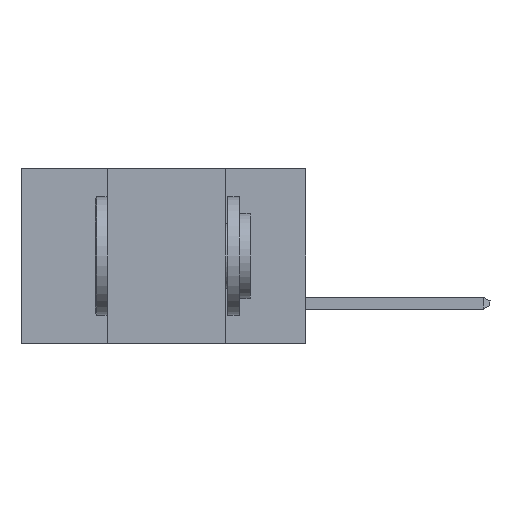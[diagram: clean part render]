
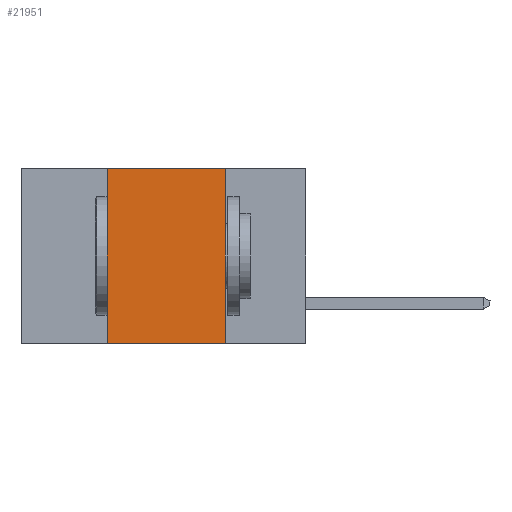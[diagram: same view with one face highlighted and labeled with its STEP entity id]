
A CAD part, left-side view. The second image highlights one B-rep face of the part: STEP entity #21951.
In plain terms, the highlighted planar face has unit normal (-1, 0, 0).
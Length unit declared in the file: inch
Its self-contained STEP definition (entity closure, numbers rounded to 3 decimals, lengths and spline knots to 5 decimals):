
#622 = LINE ( 'NONE', #13256, #5973 ) ;
#3241 = CARTESIAN_POINT ( 'NONE',  ( 0., 0.6, -0.37 ) ) ;
#3280 = EDGE_CURVE ( 'NONE', #24611, #7373, #12283, .T. ) ;
#3740 = CARTESIAN_POINT ( 'NONE',  ( 0., 0.42, -0.37 ) ) ;
#4066 = ORIENTED_EDGE ( 'NONE', *, *, #8670, .T. ) ;
#4547 = CARTESIAN_POINT ( 'NONE',  ( 0., 0.6, 0. ) ) ;
#5973 = VECTOR ( 'NONE', #11085, 39.37008 ) ;
#7336 = VECTOR ( 'NONE', #20811, 39.37008 ) ;
#7368 = CARTESIAN_POINT ( 'NONE',  ( 0., 0.17, -0.37 ) ) ;
#7373 = VERTEX_POINT ( 'NONE', #23233 ) ;
#7678 = DIRECTION ( 'NONE',  ( 0., 0., 1. ) ) ;
#8017 = FACE_OUTER_BOUND ( 'NONE', #8884, .T. ) ;
#8667 = ORIENTED_EDGE ( 'NONE', *, *, #25866, .F. ) ;
#8670 = EDGE_CURVE ( 'NONE', #24611, #18544, #21318, .T. ) ;
#8884 = EDGE_LOOP ( 'NONE', ( #8667, #12462, #17641, #4066 ) ) ;
#10656 = DIRECTION ( 'NONE',  ( 0., 0., -1. ) ) ;
#11085 = DIRECTION ( 'NONE',  ( 0., 0., -1. ) ) ;
#12283 = LINE ( 'NONE', #25920, #23693 ) ;
#12462 = ORIENTED_EDGE ( 'NONE', *, *, #21655, .F. ) ;
#12603 = PLANE ( 'NONE',  #24727 ) ;
#12743 = VECTOR ( 'NONE', #26373, 39.37008 ) ;
#13256 = CARTESIAN_POINT ( 'NONE',  ( 0., 0.17, 0. ) ) ;
#17641 = ORIENTED_EDGE ( 'NONE', *, *, #3280, .F. ) ;
#18544 = VERTEX_POINT ( 'NONE', #7368 ) ;
#19213 = VERTEX_POINT ( 'NONE', #20137 ) ;
#20137 = CARTESIAN_POINT ( 'NONE',  ( 0., 0.17, 0. ) ) ;
#20811 = DIRECTION ( 'NONE',  ( 0., -1., 0. ) ) ;
#21318 = LINE ( 'NONE', #3241, #12743 ) ;
#21655 = EDGE_CURVE ( 'NONE', #7373, #19213, #24424, .T. ) ;
#21951 = ADVANCED_FACE ( 'NONE', ( #8017 ), #12603, .F. ) ;
#23233 = CARTESIAN_POINT ( 'NONE',  ( 0., 0.42, 0. ) ) ;
#23693 = VECTOR ( 'NONE', #7678, 39.37008 ) ;
#24424 = LINE ( 'NONE', #4547, #7336 ) ;
#24611 = VERTEX_POINT ( 'NONE', #3740 ) ;
#24727 = AXIS2_PLACEMENT_3D ( 'NONE', #28239, #28736, #10656 ) ;
#25866 = EDGE_CURVE ( 'NONE', #19213, #18544, #622, .T. ) ;
#25920 = CARTESIAN_POINT ( 'NONE',  ( 0., 0.42, 0. ) ) ;
#26373 = DIRECTION ( 'NONE',  ( 0., -1., 0. ) ) ;
#28239 = CARTESIAN_POINT ( 'NONE',  ( 0., 0.6, 0. ) ) ;
#28736 = DIRECTION ( 'NONE',  ( 1., 0., 0. ) ) ;
